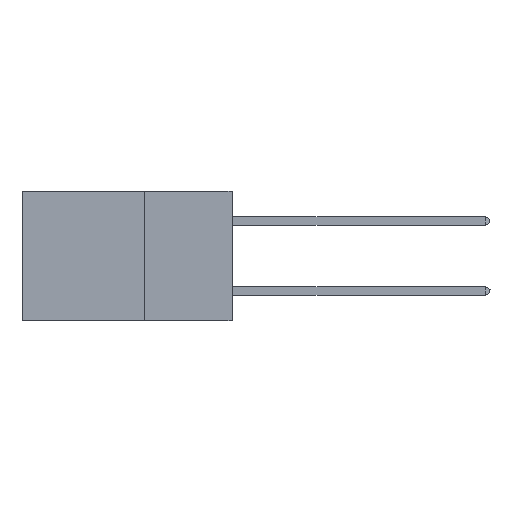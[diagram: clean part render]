
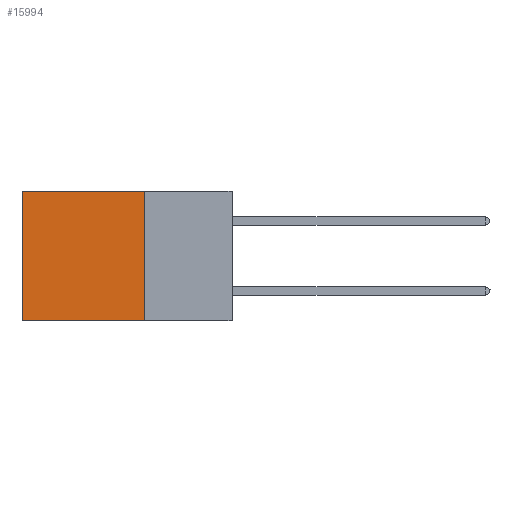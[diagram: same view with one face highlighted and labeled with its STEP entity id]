
A CAD part, left-side view. The second image highlights one B-rep face of the part: STEP entity #15994.
In plain terms, the highlighted planar face has unit normal (-1, 0, 0).
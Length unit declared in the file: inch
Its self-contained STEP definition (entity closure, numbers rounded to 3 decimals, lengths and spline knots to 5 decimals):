
#766 = CARTESIAN_POINT ( 'NONE',  ( 0.2875, 0.25, 0. ) ) ;
#2517 = VECTOR ( 'NONE', #15018, 39.37008 ) ;
#3189 = CARTESIAN_POINT ( 'NONE',  ( 0.2875, 0.6, -0.37 ) ) ;
#3191 = DIRECTION ( 'NONE',  ( 0., 0., -1. ) ) ;
#3869 = FACE_OUTER_BOUND ( 'NONE', #13974, .T. ) ;
#4323 = ORIENTED_EDGE ( 'NONE', *, *, #17690, .F. ) ;
#4598 = VERTEX_POINT ( 'NONE', #10971 ) ;
#4852 = AXIS2_PLACEMENT_3D ( 'NONE', #7768, #30337, #15218 ) ;
#5214 = VERTEX_POINT ( 'NONE', #3189 ) ;
#5346 = VERTEX_POINT ( 'NONE', #30477 ) ;
#5984 = LINE ( 'NONE', #26249, #29507 ) ;
#6740 = DIRECTION ( 'NONE',  ( 0., 1., 0. ) ) ;
#6907 = VECTOR ( 'NONE', #18635, 39.37008 ) ;
#7693 = LINE ( 'NONE', #11129, #6907 ) ;
#7768 = CARTESIAN_POINT ( 'NONE',  ( 0.2875, 0.25, 0. ) ) ;
#9300 = VERTEX_POINT ( 'NONE', #766 ) ;
#10971 = CARTESIAN_POINT ( 'NONE',  ( 0.2875, 0.6, 0. ) ) ;
#11129 = CARTESIAN_POINT ( 'NONE',  ( 0.2875, 0.25, -0.37 ) ) ;
#13946 = CARTESIAN_POINT ( 'NONE',  ( 0.2875, 0.25, 0. ) ) ;
#13974 = EDGE_LOOP ( 'NONE', ( #20642, #24598, #4323, #18505 ) ) ;
#15018 = DIRECTION ( 'NONE',  ( 0., 0., -1. ) ) ;
#15218 = DIRECTION ( 'NONE',  ( 0., 0., -1. ) ) ;
#15994 = ADVANCED_FACE ( 'NONE', ( #3869 ), #17833, .F. ) ;
#17690 = EDGE_CURVE ( 'NONE', #9300, #5346, #22821, .T. ) ;
#17833 = PLANE ( 'NONE',  #4852 ) ;
#18505 = ORIENTED_EDGE ( 'NONE', *, *, #22536, .T. ) ;
#18635 = DIRECTION ( 'NONE',  ( 0., 1., 0. ) ) ;
#19264 = EDGE_CURVE ( 'NONE', #4598, #5214, #5984, .T. ) ;
#20642 = ORIENTED_EDGE ( 'NONE', *, *, #19264, .T. ) ;
#21673 = CARTESIAN_POINT ( 'NONE',  ( 0.2875, 0.25, 0. ) ) ;
#22536 = EDGE_CURVE ( 'NONE', #9300, #4598, #28092, .T. ) ;
#22821 = LINE ( 'NONE', #13946, #2517 ) ;
#24598 = ORIENTED_EDGE ( 'NONE', *, *, #26180, .F. ) ;
#26180 = EDGE_CURVE ( 'NONE', #5346, #5214, #7693, .T. ) ;
#26249 = CARTESIAN_POINT ( 'NONE',  ( 0.2875, 0.6, 0. ) ) ;
#28092 = LINE ( 'NONE', #21673, #31678 ) ;
#29507 = VECTOR ( 'NONE', #3191, 39.37008 ) ;
#30337 = DIRECTION ( 'NONE',  ( 1., 0., 0. ) ) ;
#30477 = CARTESIAN_POINT ( 'NONE',  ( 0.2875, 0.25, -0.37 ) ) ;
#31678 = VECTOR ( 'NONE', #6740, 39.37008 ) ;
